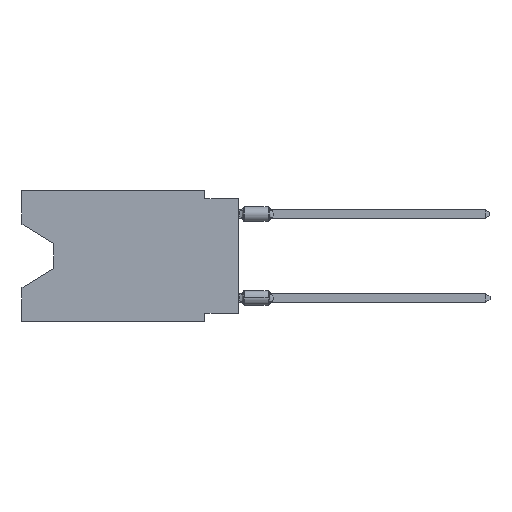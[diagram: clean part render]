
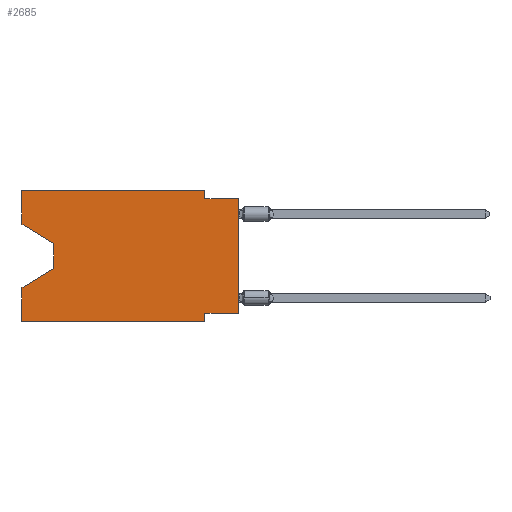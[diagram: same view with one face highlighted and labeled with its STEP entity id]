
A CAD part, left-side view. The second image highlights one B-rep face of the part: STEP entity #2685.
In plain terms, the highlighted planar face has unit normal (-1, 0, 0).
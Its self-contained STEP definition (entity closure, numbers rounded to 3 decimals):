
#310 = LINE ( 'NONE', #8966, #8546 ) ;
#359 = CARTESIAN_POINT ( 'NONE',  ( 0., 0., -9.271 ) ) ;
#543 = CARTESIAN_POINT ( 'NONE',  ( 0., 2.54, -9.271 ) ) ;
#599 = DIRECTION ( 'NONE',  ( 0., 0., -1. ) ) ;
#816 = DIRECTION ( 'NONE',  ( 0., 0., 1. ) ) ;
#823 = DIRECTION ( 'NONE',  ( 0., 0., 1. ) ) ;
#1161 = LINE ( 'NONE', #22145, #4838 ) ;
#1223 = VECTOR ( 'NONE', #5884, 1000. ) ;
#1804 = VERTEX_POINT ( 'NONE', #17719 ) ;
#1905 = CARTESIAN_POINT ( 'NONE',  ( 0., 2.54, -9.906 ) ) ;
#1991 = CARTESIAN_POINT ( 'NONE',  ( 0., 0., 0. ) ) ;
#2562 = CARTESIAN_POINT ( 'NONE',  ( 0., 16.383, 0. ) ) ;
#2685 = ADVANCED_FACE ( 'NONE', ( #18008 ), #13155, .F. ) ;
#2720 = EDGE_CURVE ( 'NONE', #16590, #16013, #21457, .T. ) ;
#2763 = EDGE_CURVE ( 'NONE', #13049, #14908, #16283, .T. ) ;
#3714 = CARTESIAN_POINT ( 'NONE',  ( 0., 16.383, -7.36 ) ) ;
#4012 = EDGE_CURVE ( 'NONE', #12585, #8322, #1161, .T. ) ;
#4024 = VECTOR ( 'NONE', #823, 1000. ) ;
#4300 = LINE ( 'NONE', #11104, #4024 ) ;
#4451 = VECTOR ( 'NONE', #15985, 1000. ) ;
#4838 = VECTOR ( 'NONE', #14896, 1000. ) ;
#5123 = LINE ( 'NONE', #10205, #19905 ) ;
#5884 = DIRECTION ( 'NONE',  ( 0., -1., 0. ) ) ;
#5976 = EDGE_CURVE ( 'NONE', #16590, #12031, #310, .T. ) ;
#6113 = VERTEX_POINT ( 'NONE', #10002 ) ;
#6547 = LINE ( 'NONE', #13551, #11023 ) ;
#6690 = ORIENTED_EDGE ( 'NONE', *, *, #17645, .T. ) ;
#6799 = VECTOR ( 'NONE', #14891, 1000. ) ;
#6942 = CARTESIAN_POINT ( 'NONE',  ( 0., 16.383, 0. ) ) ;
#7091 = VECTOR ( 'NONE', #599, 1000. ) ;
#7462 = ORIENTED_EDGE ( 'NONE', *, *, #4012, .T. ) ;
#7546 = AXIS2_PLACEMENT_3D ( 'NONE', #2562, #13040, #14556 ) ;
#8322 = VERTEX_POINT ( 'NONE', #9085 ) ;
#8518 = ORIENTED_EDGE ( 'NONE', *, *, #2720, .F. ) ;
#8546 = VECTOR ( 'NONE', #9441, 1000. ) ;
#8966 = CARTESIAN_POINT ( 'NONE',  ( 0., 16.383, -9.906 ) ) ;
#9085 = CARTESIAN_POINT ( 'NONE',  ( 0., 13.97, -4.013 ) ) ;
#9441 = DIRECTION ( 'NONE',  ( 0., -1., 0. ) ) ;
#9579 = ORIENTED_EDGE ( 'NONE', *, *, #16060, .F. ) ;
#9721 = EDGE_CURVE ( 'NONE', #1804, #16013, #20929, .T. ) ;
#9910 = EDGE_CURVE ( 'NONE', #14908, #12031, #17711, .T. ) ;
#10002 = CARTESIAN_POINT ( 'NONE',  ( 0., 0., -0.635 ) ) ;
#10205 = CARTESIAN_POINT ( 'NONE',  ( 0., 13.97, -4.013 ) ) ;
#10348 = CARTESIAN_POINT ( 'NONE',  ( 0., 13.97, -5.893 ) ) ;
#10987 = ORIENTED_EDGE ( 'NONE', *, *, #16031, .F. ) ;
#11017 = ORIENTED_EDGE ( 'NONE', *, *, #9721, .T. ) ;
#11023 = VECTOR ( 'NONE', #20585, 1000. ) ;
#11065 = LINE ( 'NONE', #21660, #1223 ) ;
#11104 = CARTESIAN_POINT ( 'NONE',  ( 0., 16.383, 0. ) ) ;
#11815 = DIRECTION ( 'NONE',  ( 0., 0., -1. ) ) ;
#12031 = VERTEX_POINT ( 'NONE', #14399 ) ;
#12098 = ORIENTED_EDGE ( 'NONE', *, *, #13371, .F. ) ;
#12148 = VECTOR ( 'NONE', #20704, 1000. ) ;
#12318 = VECTOR ( 'NONE', #816, 1000. ) ;
#12585 = VERTEX_POINT ( 'NONE', #18952 ) ;
#12705 = CARTESIAN_POINT ( 'NONE',  ( 0., 2.54, 0. ) ) ;
#13040 = DIRECTION ( 'NONE',  ( 1., 0., 0. ) ) ;
#13049 = VERTEX_POINT ( 'NONE', #14890 ) ;
#13155 = PLANE ( 'NONE',  #7546 ) ;
#13371 = EDGE_CURVE ( 'NONE', #21890, #6113, #11065, .T. ) ;
#13551 = CARTESIAN_POINT ( 'NONE',  ( 0., 16.383, 0. ) ) ;
#14323 = VERTEX_POINT ( 'NONE', #6942 ) ;
#14399 = CARTESIAN_POINT ( 'NONE',  ( 0., 2.54, -9.906 ) ) ;
#14417 = ORIENTED_EDGE ( 'NONE', *, *, #18850, .F. ) ;
#14556 = DIRECTION ( 'NONE',  ( 0., 0., -1. ) ) ;
#14570 = DIRECTION ( 'NONE',  ( 0., 0., 1. ) ) ;
#14890 = CARTESIAN_POINT ( 'NONE',  ( 0., 0., -9.271 ) ) ;
#14891 = DIRECTION ( 'NONE',  ( 0., 1., 0. ) ) ;
#14896 = DIRECTION ( 'NONE',  ( 0., -0.855, -0.519 ) ) ;
#14908 = VERTEX_POINT ( 'NONE', #543 ) ;
#15874 = VECTOR ( 'NONE', #14570, 1000. ) ;
#15985 = DIRECTION ( 'NONE',  ( 0., 0., -1. ) ) ;
#16013 = VERTEX_POINT ( 'NONE', #3714 ) ;
#16031 = EDGE_CURVE ( 'NONE', #14323, #22361, #6547, .T. ) ;
#16060 = EDGE_CURVE ( 'NONE', #12585, #14323, #4300, .T. ) ;
#16223 = ORIENTED_EDGE ( 'NONE', *, *, #9910, .F. ) ;
#16283 = LINE ( 'NONE', #359, #6799 ) ;
#16528 = LINE ( 'NONE', #12705, #7091 ) ;
#16590 = VERTEX_POINT ( 'NONE', #19601 ) ;
#16635 = CARTESIAN_POINT ( 'NONE',  ( 0., 16.383, 0. ) ) ;
#17645 = EDGE_CURVE ( 'NONE', #8322, #1804, #5123, .T. ) ;
#17711 = LINE ( 'NONE', #1905, #4451 ) ;
#17719 = CARTESIAN_POINT ( 'NONE',  ( 0., 13.97, -5.893 ) ) ;
#17755 = EDGE_CURVE ( 'NONE', #13049, #6113, #18021, .T. ) ;
#18008 = FACE_OUTER_BOUND ( 'NONE', #19646, .T. ) ;
#18016 = ORIENTED_EDGE ( 'NONE', *, *, #5976, .T. ) ;
#18021 = LINE ( 'NONE', #1991, #15874 ) ;
#18325 = CARTESIAN_POINT ( 'NONE',  ( 0., 2.54, 0. ) ) ;
#18850 = EDGE_CURVE ( 'NONE', #22361, #21890, #16528, .T. ) ;
#18952 = CARTESIAN_POINT ( 'NONE',  ( 0., 16.383, -2.546 ) ) ;
#19211 = ORIENTED_EDGE ( 'NONE', *, *, #2763, .F. ) ;
#19285 = CARTESIAN_POINT ( 'NONE',  ( 0., 2.54, -0.635 ) ) ;
#19601 = CARTESIAN_POINT ( 'NONE',  ( 0., 16.383, -9.906 ) ) ;
#19646 = EDGE_LOOP ( 'NONE', ( #7462, #6690, #11017, #8518, #18016, #16223, #19211, #20154, #12098, #14417, #10987, #9579 ) ) ;
#19905 = VECTOR ( 'NONE', #11815, 1000. ) ;
#20154 = ORIENTED_EDGE ( 'NONE', *, *, #17755, .T. ) ;
#20585 = DIRECTION ( 'NONE',  ( 0., -1., 0. ) ) ;
#20704 = DIRECTION ( 'NONE',  ( 0., 0.855, -0.519 ) ) ;
#20929 = LINE ( 'NONE', #10348, #12148 ) ;
#21457 = LINE ( 'NONE', #16635, #12318 ) ;
#21660 = CARTESIAN_POINT ( 'NONE',  ( 0., 0., -0.635 ) ) ;
#21890 = VERTEX_POINT ( 'NONE', #19285 ) ;
#22145 = CARTESIAN_POINT ( 'NONE',  ( 0., 16.383, -2.546 ) ) ;
#22361 = VERTEX_POINT ( 'NONE', #18325 ) ;
